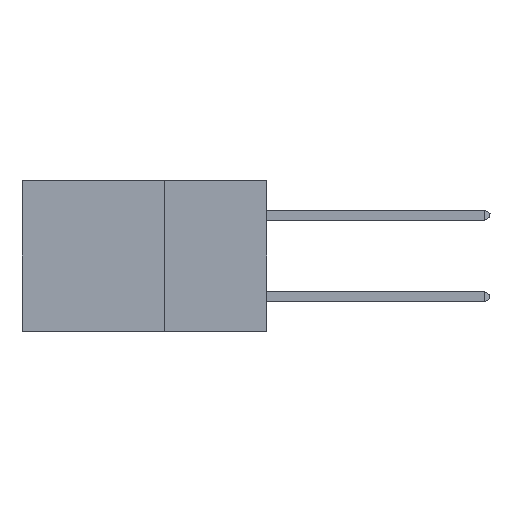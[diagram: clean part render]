
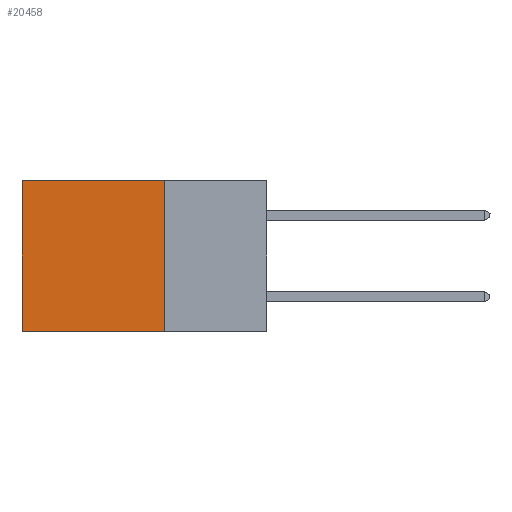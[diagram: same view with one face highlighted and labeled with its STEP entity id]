
A CAD part, left-side view. The second image highlights one B-rep face of the part: STEP entity #20458.
In plain terms, the highlighted planar face has unit normal (-1, 0, 0).
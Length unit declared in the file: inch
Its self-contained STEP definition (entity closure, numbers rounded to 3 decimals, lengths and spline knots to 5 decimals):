
#43 = CARTESIAN_POINT ( 'NONE',  ( 0.2875, 0.6, 0. ) ) ;
#1269 = AXIS2_PLACEMENT_3D ( 'NONE', #9240, #14799, #22298 ) ;
#1662 = VERTEX_POINT ( 'NONE', #14955 ) ;
#1942 = EDGE_CURVE ( 'NONE', #2639, #13328, #5233, .T. ) ;
#1999 = FACE_OUTER_BOUND ( 'NONE', #4268, .T. ) ;
#2634 = ORIENTED_EDGE ( 'NONE', *, *, #16984, .T. ) ;
#2639 = VERTEX_POINT ( 'NONE', #7754 ) ;
#2969 = VERTEX_POINT ( 'NONE', #23045 ) ;
#2991 = LINE ( 'NONE', #18237, #18806 ) ;
#4268 = EDGE_LOOP ( 'NONE', ( #2634, #11914, #5909, #11248 ) ) ;
#4523 = VECTOR ( 'NONE', #12712, 39.37008 ) ;
#4832 = CARTESIAN_POINT ( 'NONE',  ( 0.2875, 0.25, -0.37 ) ) ;
#5233 = LINE ( 'NONE', #18145, #4523 ) ;
#5529 = LINE ( 'NONE', #4832, #22482 ) ;
#5909 = ORIENTED_EDGE ( 'NONE', *, *, #14940, .F. ) ;
#7754 = CARTESIAN_POINT ( 'NONE',  ( 0.2875, 0.25, 0. ) ) ;
#9240 = CARTESIAN_POINT ( 'NONE',  ( 0.2875, 0.25, 0. ) ) ;
#9481 = PLANE ( 'NONE',  #1269 ) ;
#11248 = ORIENTED_EDGE ( 'NONE', *, *, #1942, .T. ) ;
#11914 = ORIENTED_EDGE ( 'NONE', *, *, #20781, .F. ) ;
#12571 = DIRECTION ( 'NONE',  ( 0., 0., -1. ) ) ;
#12712 = DIRECTION ( 'NONE',  ( 0., 1., 0. ) ) ;
#13015 = DIRECTION ( 'NONE',  ( 0., 1., 0. ) ) ;
#13328 = VERTEX_POINT ( 'NONE', #43 ) ;
#13392 = DIRECTION ( 'NONE',  ( 0., 0., -1. ) ) ;
#14799 = DIRECTION ( 'NONE',  ( 1., 0., 0. ) ) ;
#14940 = EDGE_CURVE ( 'NONE', #2639, #2969, #2991, .T. ) ;
#14955 = CARTESIAN_POINT ( 'NONE',  ( 0.2875, 0.6, -0.37 ) ) ;
#16984 = EDGE_CURVE ( 'NONE', #13328, #1662, #18931, .T. ) ;
#18145 = CARTESIAN_POINT ( 'NONE',  ( 0.2875, 0.25, 0. ) ) ;
#18237 = CARTESIAN_POINT ( 'NONE',  ( 0.2875, 0.25, 0. ) ) ;
#18806 = VECTOR ( 'NONE', #12571, 39.37008 ) ;
#18931 = LINE ( 'NONE', #19172, #20069 ) ;
#19172 = CARTESIAN_POINT ( 'NONE',  ( 0.2875, 0.6, 0. ) ) ;
#20069 = VECTOR ( 'NONE', #13392, 39.37008 ) ;
#20458 = ADVANCED_FACE ( 'NONE', ( #1999 ), #9481, .F. ) ;
#20781 = EDGE_CURVE ( 'NONE', #2969, #1662, #5529, .T. ) ;
#22298 = DIRECTION ( 'NONE',  ( 0., 0., -1. ) ) ;
#22482 = VECTOR ( 'NONE', #13015, 39.37008 ) ;
#23045 = CARTESIAN_POINT ( 'NONE',  ( 0.2875, 0.25, -0.37 ) ) ;
